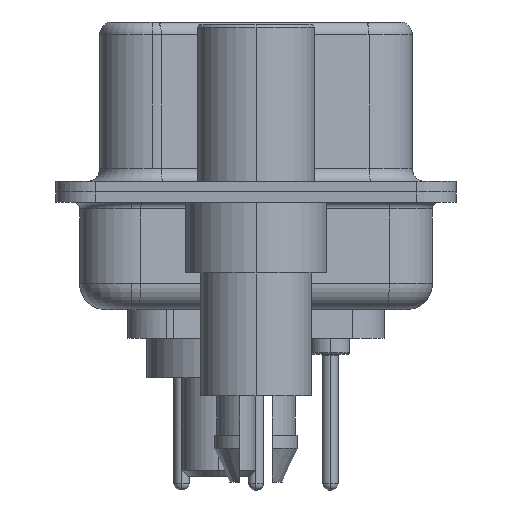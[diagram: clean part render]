
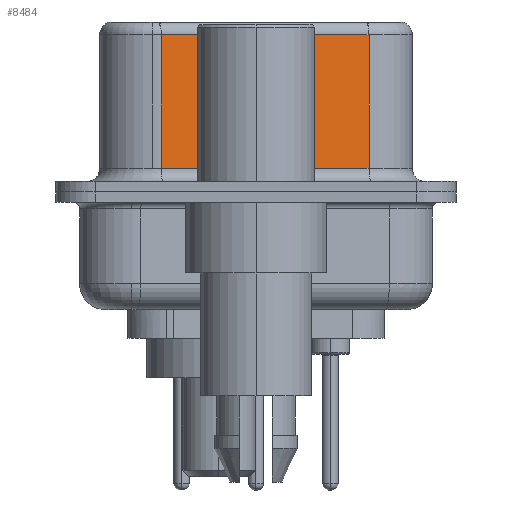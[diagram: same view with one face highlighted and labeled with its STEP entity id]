
A CAD part, left-side view. The second image highlights one B-rep face of the part: STEP entity #8484.
In plain terms, the highlighted planar face has unit normal (-0.985, -0.174, 0).
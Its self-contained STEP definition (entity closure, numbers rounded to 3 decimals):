
#1808 = DIRECTION ( 'NONE',  ( 0., 0., -1. ) ) ;
#1872 = VERTEX_POINT ( 'NONE', #3781 ) ;
#2426 = ORIENTED_EDGE ( 'NONE', *, *, #23202, .T. ) ;
#2584 = DIRECTION ( 'NONE',  ( -0.174, 0.985, 0. ) ) ;
#2645 = ORIENTED_EDGE ( 'NONE', *, *, #17760, .T. ) ;
#2912 = FACE_OUTER_BOUND ( 'NONE', #18840, .T. ) ;
#3019 = VECTOR ( 'NONE', #8543, 1000. ) ;
#3743 = PLANE ( 'NONE',  #4134 ) ;
#3781 = CARTESIAN_POINT ( 'NONE',  ( 5.132, -4.322, 0.9 ) ) ;
#4134 = AXIS2_PLACEMENT_3D ( 'NONE', #5668, #4550, #2584 ) ;
#4550 = DIRECTION ( 'NONE',  ( 0.985, 0.174, 0. ) ) ;
#4970 = LINE ( 'NONE', #22258, #16448 ) ;
#5343 = CARTESIAN_POINT ( 'NONE',  ( 3.73, 3.628, 0.9 ) ) ;
#5471 = VECTOR ( 'NONE', #1808, 1000. ) ;
#5668 = CARTESIAN_POINT ( 'NONE',  ( 5.132, -4.322, 6.52 ) ) ;
#6205 = VERTEX_POINT ( 'NONE', #25491 ) ;
#6573 = ORIENTED_EDGE ( 'NONE', *, *, #18782, .F. ) ;
#8438 = LINE ( 'NONE', #13126, #3019 ) ;
#8484 = ADVANCED_FACE ( 'NONE', ( #2912 ), #3743, .F. ) ;
#8543 = DIRECTION ( 'NONE',  ( -0.174, 0.985, 0. ) ) ;
#11340 = DIRECTION ( 'NONE',  ( 0., 0., -1. ) ) ;
#11566 = LINE ( 'NONE', #17903, #5471 ) ;
#12594 = EDGE_CURVE ( 'NONE', #24584, #1872, #4970, .T. ) ;
#13126 = CARTESIAN_POINT ( 'NONE',  ( 5.132, -4.322, 6.02 ) ) ;
#13523 = CARTESIAN_POINT ( 'NONE',  ( 5.132, -4.322, 6.52 ) ) ;
#16359 = ORIENTED_EDGE ( 'NONE', *, *, #12594, .T. ) ;
#16448 = VECTOR ( 'NONE', #17602, 1000. ) ;
#17602 = DIRECTION ( 'NONE',  ( 0.174, -0.985, 0. ) ) ;
#17760 = EDGE_CURVE ( 'NONE', #21430, #24584, #11566, .T. ) ;
#17903 = CARTESIAN_POINT ( 'NONE',  ( 3.73, 3.628, 6.52 ) ) ;
#18782 = EDGE_CURVE ( 'NONE', #6205, #1872, #20122, .T. ) ;
#18840 = EDGE_LOOP ( 'NONE', ( #6573, #2426, #2645, #16359 ) ) ;
#19395 = VECTOR ( 'NONE', #11340, 1000. ) ;
#20122 = LINE ( 'NONE', #13523, #19395 ) ;
#21430 = VERTEX_POINT ( 'NONE', #27766 ) ;
#22258 = CARTESIAN_POINT ( 'NONE',  ( 5.132, -4.322, 0.9 ) ) ;
#23202 = EDGE_CURVE ( 'NONE', #6205, #21430, #8438, .T. ) ;
#24584 = VERTEX_POINT ( 'NONE', #5343 ) ;
#25491 = CARTESIAN_POINT ( 'NONE',  ( 5.132, -4.322, 6.02 ) ) ;
#27766 = CARTESIAN_POINT ( 'NONE',  ( 3.73, 3.628, 6.02 ) ) ;
